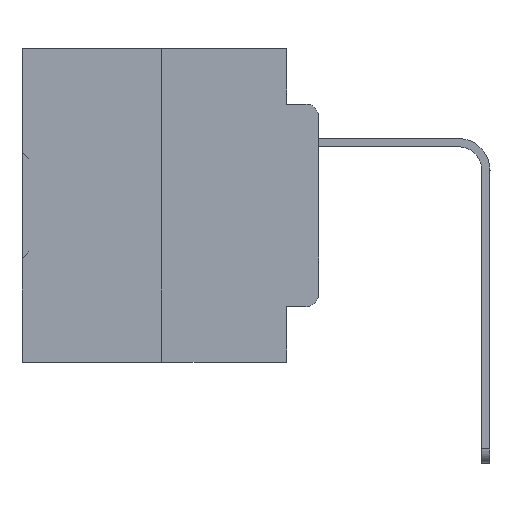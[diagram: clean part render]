
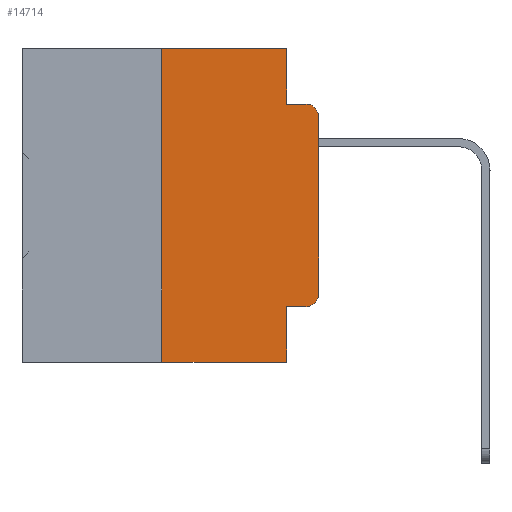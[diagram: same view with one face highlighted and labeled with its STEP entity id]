
A CAD part, left-side view. The second image highlights one B-rep face of the part: STEP entity #14714.
In plain terms, the highlighted planar face has unit normal (-1, 0, 0).
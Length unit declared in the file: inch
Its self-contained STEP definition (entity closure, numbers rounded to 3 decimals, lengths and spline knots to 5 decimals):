
#271 = CARTESIAN_POINT ( 'NONE',  ( 0., 0.02, -0.1085 ) ) ;
#587 = EDGE_CURVE ( 'NONE', #1463, #35819, #23293, .T. ) ;
#753 = LINE ( 'NONE', #22201, #30738 ) ;
#882 = DIRECTION ( 'NONE',  ( 0., 0., -1. ) ) ;
#1003 = EDGE_CURVE ( 'NONE', #38594, #35819, #18113, .T. ) ;
#1463 = VERTEX_POINT ( 'NONE', #37744 ) ;
#1948 = CARTESIAN_POINT ( 'NONE',  ( 0., 0.051, 0. ) ) ;
#2548 = CARTESIAN_POINT ( 'NONE',  ( 0., 0.051, 0. ) ) ;
#2770 = ORIENTED_EDGE ( 'NONE', *, *, #19936, .F. ) ;
#2942 = EDGE_LOOP ( 'NONE', ( #31519, #13422, #36231, #21353, #2770, #12776, #29568, #28752, #18343, #14099 ) ) ;
#3962 = CARTESIAN_POINT ( 'NONE',  ( 0., 0.473, 0. ) ) ;
#4698 = AXIS2_PLACEMENT_3D ( 'NONE', #21449, #18441, #882 ) ;
#5110 = CARTESIAN_POINT ( 'NONE',  ( 0., 0.051, -0.4115 ) ) ;
#5417 = VECTOR ( 'NONE', #12045, 39.37008 ) ;
#6144 = EDGE_CURVE ( 'NONE', #38594, #9668, #12778, .T. ) ;
#7629 = DIRECTION ( 'NONE',  ( 0., 0., -1. ) ) ;
#7797 = VECTOR ( 'NONE', #14125, 39.37008 ) ;
#9628 = LINE ( 'NONE', #30774, #16671 ) ;
#9668 = VERTEX_POINT ( 'NONE', #14737 ) ;
#10348 = CARTESIAN_POINT ( 'NONE',  ( 0., 0., -0.1085 ) ) ;
#10385 = EDGE_CURVE ( 'NONE', #33316, #19946, #9628, .T. ) ;
#10705 = CARTESIAN_POINT ( 'NONE',  ( 0., 0.25, 0. ) ) ;
#10712 = FACE_OUTER_BOUND ( 'NONE', #2942, .T. ) ;
#11438 = CARTESIAN_POINT ( 'NONE',  ( 0., 0.051, -0.4115 ) ) ;
#11958 = EDGE_CURVE ( 'NONE', #33303, #33795, #38675, .T. ) ;
#12045 = DIRECTION ( 'NONE',  ( 0., -1., 0. ) ) ;
#12776 = ORIENTED_EDGE ( 'NONE', *, *, #30021, .F. ) ;
#12778 = LINE ( 'NONE', #11438, #27247 ) ;
#12829 = VECTOR ( 'NONE', #24911, 39.37008 ) ;
#13392 = CIRCLE ( 'NONE', #34567, 0.02 ) ;
#13422 = ORIENTED_EDGE ( 'NONE', *, *, #24132, .T. ) ;
#14099 = ORIENTED_EDGE ( 'NONE', *, *, #28627, .T. ) ;
#14125 = DIRECTION ( 'NONE',  ( 0., 0., -1. ) ) ;
#14300 = VECTOR ( 'NONE', #15725, 39.37008 ) ;
#14463 = DIRECTION ( 'NONE',  ( 0., -1., 0. ) ) ;
#14714 = ADVANCED_FACE ( 'NONE', ( #10712 ), #32443, .F. ) ;
#14737 = CARTESIAN_POINT ( 'NONE',  ( 0., 0.02, -0.4115 ) ) ;
#15725 = DIRECTION ( 'NONE',  ( 0., 0., 1. ) ) ;
#16114 = DIRECTION ( 'NONE',  ( 0., 0., 1. ) ) ;
#16267 = CARTESIAN_POINT ( 'NONE',  ( 0., 0.051, -0.5 ) ) ;
#16671 = VECTOR ( 'NONE', #16114, 39.37008 ) ;
#17164 = AXIS2_PLACEMENT_3D ( 'NONE', #23450, #20960, #35690 ) ;
#18113 = LINE ( 'NONE', #1948, #7797 ) ;
#18343 = ORIENTED_EDGE ( 'NONE', *, *, #6144, .T. ) ;
#18441 = DIRECTION ( 'NONE',  ( -1., 0., 0. ) ) ;
#18910 = LINE ( 'NONE', #3962, #12829 ) ;
#19936 = EDGE_CURVE ( 'NONE', #26078, #35394, #18910, .T. ) ;
#19946 = VERTEX_POINT ( 'NONE', #10348 ) ;
#20960 = DIRECTION ( 'NONE',  ( 1., 0., 0. ) ) ;
#21353 = ORIENTED_EDGE ( 'NONE', *, *, #29534, .F. ) ;
#21449 = CARTESIAN_POINT ( 'NONE',  ( 0., 0.02, -0.3915 ) ) ;
#22201 = CARTESIAN_POINT ( 'NONE',  ( 0., 0.051, 0. ) ) ;
#22278 = LINE ( 'NONE', #30637, #14300 ) ;
#23293 = LINE ( 'NONE', #36230, #23775 ) ;
#23450 = CARTESIAN_POINT ( 'NONE',  ( 0., 0.473, 0. ) ) ;
#23775 = VECTOR ( 'NONE', #33362, 39.37008 ) ;
#24132 = EDGE_CURVE ( 'NONE', #19946, #33795, #13392, .T. ) ;
#24911 = DIRECTION ( 'NONE',  ( 0., -1., 0. ) ) ;
#24982 = CARTESIAN_POINT ( 'NONE',  ( 0., 0.02, -0.0885 ) ) ;
#26078 = VERTEX_POINT ( 'NONE', #10705 ) ;
#26952 = DIRECTION ( 'NONE',  ( 0., 0., -1. ) ) ;
#27247 = VECTOR ( 'NONE', #14463, 39.37008 ) ;
#27321 = DIRECTION ( 'NONE',  ( -1., 0., 0. ) ) ;
#28523 = CARTESIAN_POINT ( 'NONE',  ( 0., 0.051, -0.0885 ) ) ;
#28627 = EDGE_CURVE ( 'NONE', #9668, #33316, #35567, .T. ) ;
#28752 = ORIENTED_EDGE ( 'NONE', *, *, #1003, .F. ) ;
#29534 = EDGE_CURVE ( 'NONE', #35394, #33303, #753, .T. ) ;
#29568 = ORIENTED_EDGE ( 'NONE', *, *, #587, .T. ) ;
#29976 = CARTESIAN_POINT ( 'NONE',  ( 0., 0.051, -0.0885 ) ) ;
#30021 = EDGE_CURVE ( 'NONE', #1463, #26078, #22278, .T. ) ;
#30637 = CARTESIAN_POINT ( 'NONE',  ( 0., 0.25, 0. ) ) ;
#30738 = VECTOR ( 'NONE', #7629, 39.37008 ) ;
#30774 = CARTESIAN_POINT ( 'NONE',  ( 0., 0., 0. ) ) ;
#31519 = ORIENTED_EDGE ( 'NONE', *, *, #10385, .T. ) ;
#32443 = PLANE ( 'NONE',  #17164 ) ;
#33303 = VERTEX_POINT ( 'NONE', #28523 ) ;
#33316 = VERTEX_POINT ( 'NONE', #34291 ) ;
#33362 = DIRECTION ( 'NONE',  ( 0., -1., 0. ) ) ;
#33795 = VERTEX_POINT ( 'NONE', #24982 ) ;
#34291 = CARTESIAN_POINT ( 'NONE',  ( 0., 0., -0.3915 ) ) ;
#34567 = AXIS2_PLACEMENT_3D ( 'NONE', #271, #27321, #26952 ) ;
#35394 = VERTEX_POINT ( 'NONE', #2548 ) ;
#35567 = CIRCLE ( 'NONE', #4698, 0.02 ) ;
#35690 = DIRECTION ( 'NONE',  ( 0., 0., -1. ) ) ;
#35819 = VERTEX_POINT ( 'NONE', #16267 ) ;
#36230 = CARTESIAN_POINT ( 'NONE',  ( 0., 0.473, -0.5 ) ) ;
#36231 = ORIENTED_EDGE ( 'NONE', *, *, #11958, .F. ) ;
#37744 = CARTESIAN_POINT ( 'NONE',  ( 0., 0.25, -0.5 ) ) ;
#38594 = VERTEX_POINT ( 'NONE', #5110 ) ;
#38675 = LINE ( 'NONE', #29976, #5417 ) ;
